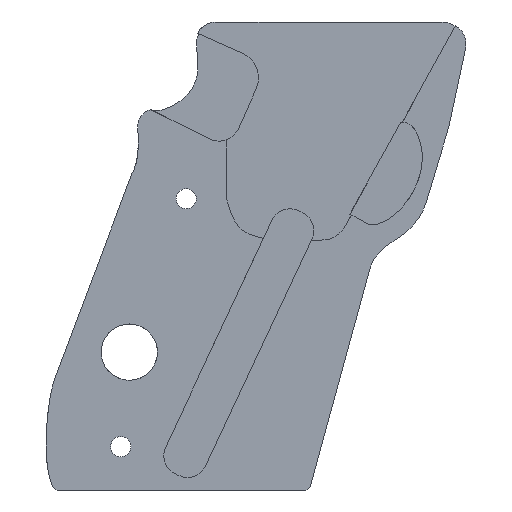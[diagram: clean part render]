
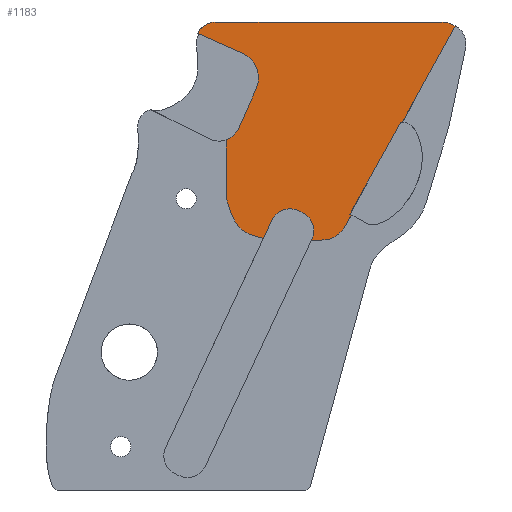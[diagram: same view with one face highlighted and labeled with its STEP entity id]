
A CAD part, front view. The second image highlights one B-rep face of the part: STEP entity #1183.
In plain terms, the highlighted planar face has unit normal (0, -1, 0).
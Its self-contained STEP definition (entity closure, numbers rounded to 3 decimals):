
#22=(
BOUNDED_CURVE()
B_SPLINE_CURVE(5,(#2917,#2918,#2919,#2920,#2921,#2922,#2923,#2924,#2925,
#2926,#2927,#2928,#2929,#2930,#2931),.UNSPECIFIED.,.F.,.F.)
B_SPLINE_CURVE_WITH_KNOTS((6,1,1,1,1,1,1,1,1,1,6),(-1.,-0.9,-0.8,-0.7,-0.6,
-0.5,-0.4,-0.3,-0.2,-0.1,0.),.UNSPECIFIED.)
CURVE()
GEOMETRIC_REPRESENTATION_ITEM()
RATIONAL_B_SPLINE_CURVE((1.,1.,1.,1.,1.,1.,1.,1.,1.,1.,1.,1.,1.,1.,1.))
REPRESENTATION_ITEM('')
);
#23=(
BOUNDED_CURVE()
B_SPLINE_CURVE(5,(#2943,#2944,#2945,#2946,#2947,#2948,#2949,#2950,#2951,
#2952,#2953,#2954,#2955,#2956,#2957),.UNSPECIFIED.,.F.,.F.)
B_SPLINE_CURVE_WITH_KNOTS((6,1,1,1,1,1,1,1,1,1,6),(-1.,-0.9,-0.8,-0.7,-0.6,
-0.5,-0.4,-0.3,-0.2,-0.1,0.),.UNSPECIFIED.)
CURVE()
GEOMETRIC_REPRESENTATION_ITEM()
RATIONAL_B_SPLINE_CURVE((1.,1.,1.,1.,1.,1.,1.,1.,1.,1.,1.,1.,1.,1.,1.))
REPRESENTATION_ITEM('')
);
#44=CIRCLE('',#1251,3.233);
#46=CIRCLE('',#1255,4.024);
#54=CIRCLE('',#1266,3.);
#55=CIRCLE('',#1267,3.);
#93=PLANE('',#1265);
#143=FACE_OUTER_BOUND('',#216,.T.);
#216=EDGE_LOOP('',(#971,#972,#973,#974,#975,#976,#977,#978,#979,#980,#981,
#982,#983,#984,#985,#986));
#291=LINE('',#2544,#374);
#294=LINE('',#2552,#377);
#303=LINE('',#2915,#386);
#304=LINE('',#2933,#387);
#305=LINE('',#2937,#388);
#306=LINE('',#2941,#389);
#307=LINE('',#2959,#390);
#308=LINE('',#2967,#391);
#374=VECTOR('',#1396,10.);
#377=VECTOR('',#1405,10.);
#386=VECTOR('',#1432,10.);
#387=VECTOR('',#1433,10.);
#388=VECTOR('',#1436,10.);
#389=VECTOR('',#1439,10.);
#390=VECTOR('',#1440,10.);
#391=VECTOR('',#1441,10.);
#464=B_SPLINE_CURVE_WITH_KNOTS('',3,(#2907,#2908,#2909,#2910,#2911,#2912,
#2913),.UNSPECIFIED.,.F.,.F.,(4,3,4),(-0.348,-0.199,
0.),.UNSPECIFIED.);
#465=B_SPLINE_CURVE_WITH_KNOTS('',3,(#2961,#2962,#2963,#2964,#2965,#2966),
 .UNSPECIFIED.,.F.,.F.,(4,2,4),(-0.605,-0.49,-0.377),
 .UNSPECIFIED.);
#537=VERTEX_POINT('',#2536);
#538=VERTEX_POINT('',#2538);
#539=VERTEX_POINT('',#2543);
#540=VERTEX_POINT('',#2547);
#541=VERTEX_POINT('',#2551);
#561=VERTEX_POINT('',#2906);
#562=VERTEX_POINT('',#2914);
#563=VERTEX_POINT('',#2916);
#564=VERTEX_POINT('',#2932);
#565=VERTEX_POINT('',#2934);
#566=VERTEX_POINT('',#2936);
#567=VERTEX_POINT('',#2938);
#568=VERTEX_POINT('',#2940);
#569=VERTEX_POINT('',#2942);
#570=VERTEX_POINT('',#2958);
#571=VERTEX_POINT('',#2960);
#677=EDGE_CURVE('',#537,#538,#44,.T.);
#680=EDGE_CURVE('',#538,#539,#291,.T.);
#682=EDGE_CURVE('',#539,#540,#46,.T.);
#684=EDGE_CURVE('',#540,#541,#294,.T.);
#714=EDGE_CURVE('',#541,#561,#464,.T.);
#715=EDGE_CURVE('',#562,#537,#303,.T.);
#716=EDGE_CURVE('',#563,#562,#22,.T.);
#717=EDGE_CURVE('',#564,#563,#304,.T.);
#718=EDGE_CURVE('',#565,#564,#54,.T.);
#719=EDGE_CURVE('',#566,#565,#305,.T.);
#720=EDGE_CURVE('',#567,#566,#55,.T.);
#721=EDGE_CURVE('',#568,#567,#306,.T.);
#722=EDGE_CURVE('',#569,#568,#23,.T.);
#723=EDGE_CURVE('',#570,#569,#307,.T.);
#724=EDGE_CURVE('',#571,#570,#465,.T.);
#725=EDGE_CURVE('',#561,#571,#308,.T.);
#971=ORIENTED_EDGE('',*,*,#714,.F.);
#972=ORIENTED_EDGE('',*,*,#684,.F.);
#973=ORIENTED_EDGE('',*,*,#682,.F.);
#974=ORIENTED_EDGE('',*,*,#680,.F.);
#975=ORIENTED_EDGE('',*,*,#677,.F.);
#976=ORIENTED_EDGE('',*,*,#715,.F.);
#977=ORIENTED_EDGE('',*,*,#716,.F.);
#978=ORIENTED_EDGE('',*,*,#717,.F.);
#979=ORIENTED_EDGE('',*,*,#718,.F.);
#980=ORIENTED_EDGE('',*,*,#719,.F.);
#981=ORIENTED_EDGE('',*,*,#720,.F.);
#982=ORIENTED_EDGE('',*,*,#721,.F.);
#983=ORIENTED_EDGE('',*,*,#722,.F.);
#984=ORIENTED_EDGE('',*,*,#723,.F.);
#985=ORIENTED_EDGE('',*,*,#724,.F.);
#986=ORIENTED_EDGE('',*,*,#725,.F.);
#1183=ADVANCED_FACE('',(#143),#93,.F.);
#1251=AXIS2_PLACEMENT_3D('',#2539,#1389,#1390);
#1255=AXIS2_PLACEMENT_3D('',#2548,#1400,#1401);
#1265=AXIS2_PLACEMENT_3D('',#2905,#1430,#1431);
#1266=AXIS2_PLACEMENT_3D('',#2935,#1434,#1435);
#1267=AXIS2_PLACEMENT_3D('',#2939,#1437,#1438);
#1389=DIRECTION('center_axis',(0.,-1.,0.));
#1390=DIRECTION('ref_axis',(0.913,0.,-0.408));
#1396=DIRECTION('',(0.408,0.,0.913));
#1400=DIRECTION('center_axis',(0.,-1.,0.));
#1401=DIRECTION('ref_axis',(0.41,0.,0.912));
#1405=DIRECTION('',(-0.912,0.,0.41));
#1430=DIRECTION('center_axis',(0.,1.,0.));
#1431=DIRECTION('ref_axis',(1.,0.,0.));
#1432=DIRECTION('',(0.,0.,1.));
#1433=DIRECTION('',(-0.424,0.,-0.906));
#1434=DIRECTION('center_axis',(0.,-1.,0.));
#1435=DIRECTION('ref_axis',(-0.906,0.,0.424));
#1436=DIRECTION('',(-0.906,0.,0.424));
#1437=DIRECTION('center_axis',(0.,-1.,0.));
#1438=DIRECTION('ref_axis',(0.424,0.,0.906));
#1439=DIRECTION('',(0.424,0.,0.906));
#1440=DIRECTION('',(-0.482,0.,-0.876));
#1441=DIRECTION('',(1.,0.,0.));
#2536=CARTESIAN_POINT('',(8.558,0.55,14.984));
#2538=CARTESIAN_POINT('',(10.423,0.55,16.71));
#2539=CARTESIAN_POINT('Origin',(7.472,0.55,18.029));
#2543=CARTESIAN_POINT('',(13.056,0.55,22.6));
#2544=CARTESIAN_POINT('',(10.423,0.55,16.71));
#2547=CARTESIAN_POINT('',(11.032,0.55,27.912));
#2548=CARTESIAN_POINT('Origin',(9.382,0.55,24.242));
#2551=CARTESIAN_POINT('',(4.309,0.55,30.935));
#2552=CARTESIAN_POINT('',(11.032,0.55,27.912));
#2905=CARTESIAN_POINT('Origin',(22.703,0.55,16.907));
#2906=CARTESIAN_POINT('',(7.172,0.55,32.594));
#2907=CARTESIAN_POINT('Ctrl Pts',(4.309,0.55,30.935));
#2908=CARTESIAN_POINT('Ctrl Pts',(4.555,0.55,31.365));
#2909=CARTESIAN_POINT('Ctrl Pts',(4.9,0.55,31.738));
#2910=CARTESIAN_POINT('Ctrl Pts',(5.308,0.55,32.018));
#2911=CARTESIAN_POINT('Ctrl Pts',(5.853,0.55,32.39));
#2912=CARTESIAN_POINT('Ctrl Pts',(6.512,0.55,32.594));
#2913=CARTESIAN_POINT('Ctrl Pts',(7.172,0.55,32.594));
#2914=CARTESIAN_POINT('',(8.558,0.55,6.483));
#2915=CARTESIAN_POINT('',(8.558,0.55,14.984));
#2916=CARTESIAN_POINT('',(14.115,0.55,0.238));
#2917=CARTESIAN_POINT('Ctrl Pts',(14.115,0.55,0.238));
#2918=CARTESIAN_POINT('Ctrl Pts',(13.94,0.55,0.284));
#2919=CARTESIAN_POINT('Ctrl Pts',(13.597,0.55,0.375));
#2920=CARTESIAN_POINT('Ctrl Pts',(13.104,0.55,0.51));
#2921=CARTESIAN_POINT('Ctrl Pts',(12.49,0.55,0.694));
#2922=CARTESIAN_POINT('Ctrl Pts',(11.793,0.55,0.966));
#2923=CARTESIAN_POINT('Ctrl Pts',(11.164,0.55,1.323));
#2924=CARTESIAN_POINT('Ctrl Pts',(10.599,0.55,1.807));
#2925=CARTESIAN_POINT('Ctrl Pts',(10.094,0.55,2.443));
#2926=CARTESIAN_POINT('Ctrl Pts',(9.642,0.55,3.232));
#2927=CARTESIAN_POINT('Ctrl Pts',(9.237,0.55,4.169));
#2928=CARTESIAN_POINT('Ctrl Pts',(8.946,0.55,5.03));
#2929=CARTESIAN_POINT('Ctrl Pts',(8.745,0.55,5.734));
#2930=CARTESIAN_POINT('Ctrl Pts',(8.619,0.55,6.229));
#2931=CARTESIAN_POINT('Ctrl Pts',(8.558,0.55,6.483));
#2932=CARTESIAN_POINT('',(15.383,0.55,2.946));
#2933=CARTESIAN_POINT('',(10.793,0.55,-6.857));
#2934=CARTESIAN_POINT('',(19.372,0.55,4.39));
#2935=CARTESIAN_POINT('Origin',(18.1,0.55,1.673));
#2936=CARTESIAN_POINT('',(19.924,0.55,4.132));
#2937=CARTESIAN_POINT('',(18.334,0.55,4.876));
#2938=CARTESIAN_POINT('',(21.369,0.55,0.143));
#2939=CARTESIAN_POINT('Origin',(18.652,0.55,1.415));
#2940=CARTESIAN_POINT('',(21.286,0.55,-0.035));
#2941=CARTESIAN_POINT('',(24.708,0.55,7.273));
#2942=CARTESIAN_POINT('',(26.317,0.55,2.057));
#2943=CARTESIAN_POINT('Ctrl Pts',(26.317,0.55,2.057));
#2944=CARTESIAN_POINT('Ctrl Pts',(26.283,0.55,1.99));
#2945=CARTESIAN_POINT('Ctrl Pts',(26.203,0.55,1.85));
#2946=CARTESIAN_POINT('Ctrl Pts',(26.045,0.55,1.62));
#2947=CARTESIAN_POINT('Ctrl Pts',(25.763,0.55,1.286));
#2948=CARTESIAN_POINT('Ctrl Pts',(25.319,0.55,0.866));
#2949=CARTESIAN_POINT('Ctrl Pts',(24.818,0.55,0.497));
#2950=CARTESIAN_POINT('Ctrl Pts',(24.289,0.55,0.226));
#2951=CARTESIAN_POINT('Ctrl Pts',(23.749,0.55,0.073));
#2952=CARTESIAN_POINT('Ctrl Pts',(23.196,0.55,0.017));
#2953=CARTESIAN_POINT('Ctrl Pts',(22.615,0.55,0.013));
#2954=CARTESIAN_POINT('Ctrl Pts',(22.115,0.55,0.014));
#2955=CARTESIAN_POINT('Ctrl Pts',(21.712,0.55,-0.002));
#2956=CARTESIAN_POINT('Ctrl Pts',(21.43,0.55,-0.023));
#2957=CARTESIAN_POINT('Ctrl Pts',(21.286,0.55,-0.035));
#2958=CARTESIAN_POINT('',(42.785,0.55,31.967));
#2959=CARTESIAN_POINT('',(26.317,0.55,2.057));
#2960=CARTESIAN_POINT('',(40.622,0.55,32.594));
#2961=CARTESIAN_POINT('Ctrl Pts',(40.622,0.55,32.594));
#2962=CARTESIAN_POINT('Ctrl Pts',(41.01,0.55,32.594));
#2963=CARTESIAN_POINT('Ctrl Pts',(41.393,0.55,32.545));
#2964=CARTESIAN_POINT('Ctrl Pts',(42.128,0.55,32.334));
#2965=CARTESIAN_POINT('Ctrl Pts',(42.472,0.55,32.177));
#2966=CARTESIAN_POINT('Ctrl Pts',(42.785,0.55,31.967));
#2967=CARTESIAN_POINT('',(8.985,0.55,32.594));
